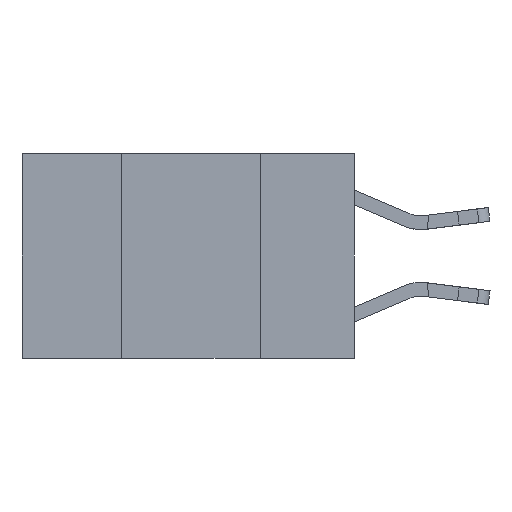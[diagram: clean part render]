
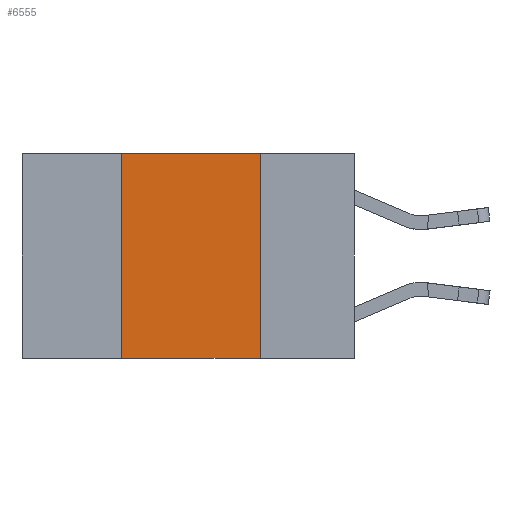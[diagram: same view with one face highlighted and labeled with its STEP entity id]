
A CAD part, left-side view. The second image highlights one B-rep face of the part: STEP entity #6555.
In plain terms, the highlighted planar face has unit normal (-1, 0, 0).
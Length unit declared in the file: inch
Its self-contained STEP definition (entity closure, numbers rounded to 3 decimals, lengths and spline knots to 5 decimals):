
#209 = AXIS2_PLACEMENT_3D ( 'NONE', #18573, #6807, #18639 ) ;
#926 = LINE ( 'NONE', #3026, #18822 ) ;
#1533 = VERTEX_POINT ( 'NONE', #4052 ) ;
#1589 = EDGE_CURVE ( 'NONE', #10909, #19178, #926, .T. ) ;
#2381 = DIRECTION ( 'NONE',  ( 0., 0., 1. ) ) ;
#3026 = CARTESIAN_POINT ( 'NONE',  ( 0., 0.42, 0. ) ) ;
#4052 = CARTESIAN_POINT ( 'NONE',  ( 0., 0.17, 0. ) ) ;
#4155 = VECTOR ( 'NONE', #7920, 39.37008 ) ;
#4959 = PLANE ( 'NONE',  #209 ) ;
#6555 = ADVANCED_FACE ( 'NONE', ( #13518 ), #4959, .F. ) ;
#6807 = DIRECTION ( 'NONE',  ( 1., 0., 0. ) ) ;
#7920 = DIRECTION ( 'NONE',  ( 0., -1., 0. ) ) ;
#8208 = VERTEX_POINT ( 'NONE', #20956 ) ;
#9042 = LINE ( 'NONE', #21302, #4155 ) ;
#10380 = EDGE_CURVE ( 'NONE', #19178, #1533, #11988, .T. ) ;
#10909 = VERTEX_POINT ( 'NONE', #15804 ) ;
#11988 = LINE ( 'NONE', #20511, #19705 ) ;
#12841 = ORIENTED_EDGE ( 'NONE', *, *, #16161, .T. ) ;
#13518 = FACE_OUTER_BOUND ( 'NONE', #16809, .T. ) ;
#14460 = CARTESIAN_POINT ( 'NONE',  ( 0., 0.17, 0. ) ) ;
#14670 = ORIENTED_EDGE ( 'NONE', *, *, #21590, .F. ) ;
#15197 = ORIENTED_EDGE ( 'NONE', *, *, #10380, .F. ) ;
#15804 = CARTESIAN_POINT ( 'NONE',  ( 0., 0.42, -0.37 ) ) ;
#16150 = DIRECTION ( 'NONE',  ( 0., 0., -1. ) ) ;
#16161 = EDGE_CURVE ( 'NONE', #10909, #8208, #9042, .T. ) ;
#16263 = ORIENTED_EDGE ( 'NONE', *, *, #1589, .F. ) ;
#16809 = EDGE_LOOP ( 'NONE', ( #14670, #15197, #16263, #12841 ) ) ;
#18573 = CARTESIAN_POINT ( 'NONE',  ( 0., 0.6, 0. ) ) ;
#18639 = DIRECTION ( 'NONE',  ( 0., 0., -1. ) ) ;
#18751 = VECTOR ( 'NONE', #16150, 39.37008 ) ;
#18822 = VECTOR ( 'NONE', #2381, 39.37008 ) ;
#19178 = VERTEX_POINT ( 'NONE', #21171 ) ;
#19252 = LINE ( 'NONE', #14460, #18751 ) ;
#19705 = VECTOR ( 'NONE', #22153, 39.37008 ) ;
#20511 = CARTESIAN_POINT ( 'NONE',  ( 0., 0.6, 0. ) ) ;
#20956 = CARTESIAN_POINT ( 'NONE',  ( 0., 0.17, -0.37 ) ) ;
#21171 = CARTESIAN_POINT ( 'NONE',  ( 0., 0.42, 0. ) ) ;
#21302 = CARTESIAN_POINT ( 'NONE',  ( 0., 0.6, -0.37 ) ) ;
#21590 = EDGE_CURVE ( 'NONE', #1533, #8208, #19252, .T. ) ;
#22153 = DIRECTION ( 'NONE',  ( 0., -1., 0. ) ) ;
